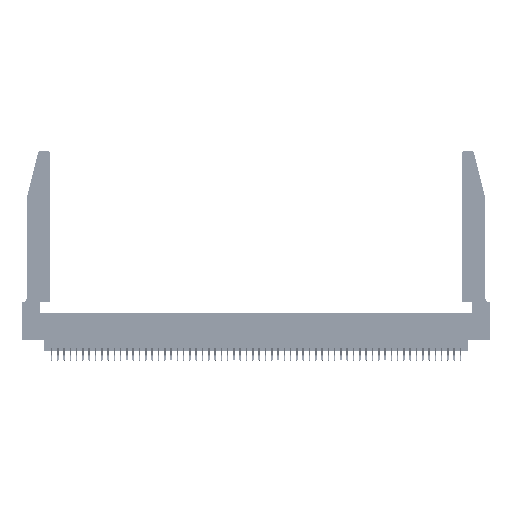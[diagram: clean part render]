
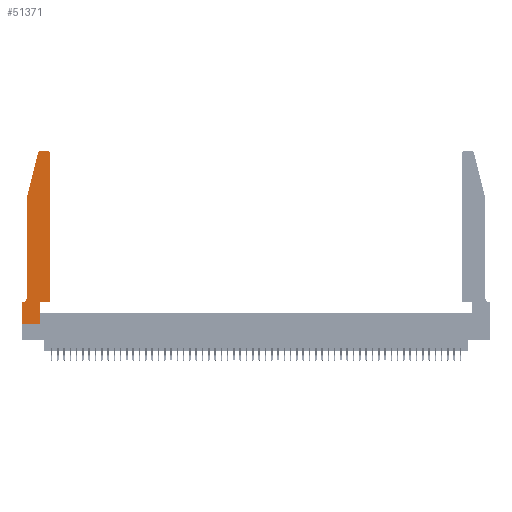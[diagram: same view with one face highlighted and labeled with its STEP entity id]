
A CAD part, top view. The second image highlights one B-rep face of the part: STEP entity #51371.
In plain terms, the highlighted planar face has unit normal (0, 0, 1).
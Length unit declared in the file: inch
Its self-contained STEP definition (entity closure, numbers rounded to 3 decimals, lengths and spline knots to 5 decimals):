
#344 = ORIENTED_EDGE ( 'NONE', *, *, #10502, .T. ) ;
#1664 = CARTESIAN_POINT ( 'NONE',  ( 0.4505, 0.35, 0.37 ) ) ;
#1841 = EDGE_CURVE ( 'NONE', #34388, #30202, #33732, .T. ) ;
#3123 = VECTOR ( 'NONE', #31397, 39.37008 ) ;
#5696 = CIRCLE ( 'NONE', #37060, 0.03 ) ;
#5752 = ORIENTED_EDGE ( 'NONE', *, *, #50961, .T. ) ;
#5858 = VECTOR ( 'NONE', #29512, 39.37008 ) ;
#6128 = CARTESIAN_POINT ( 'NONE',  ( 0.0755, 0.35, 0.37 ) ) ;
#6189 = CARTESIAN_POINT ( 'NONE',  ( 0.25487, 2.72718, 0.37 ) ) ;
#6428 = VERTEX_POINT ( 'NONE', #23156 ) ;
#8055 = DIRECTION ( 'NONE',  ( 1., 0., 0. ) ) ;
#8264 = DIRECTION ( 'NONE',  ( 0., -1., 0. ) ) ;
#8941 = CARTESIAN_POINT ( 'NONE',  ( 0.284, 2.72, 0.37 ) ) ;
#8948 = EDGE_CURVE ( 'NONE', #23391, #43217, #25297, .T. ) ;
#9113 = ORIENTED_EDGE ( 'NONE', *, *, #9363, .T. ) ;
#9363 = EDGE_CURVE ( 'NONE', #19463, #23645, #52215, .T. ) ;
#9889 = CARTESIAN_POINT ( 'NONE',  ( 0.2605, 2.75, 0.37 ) ) ;
#10220 = VECTOR ( 'NONE', #18293, 39.37008 ) ;
#10400 = DIRECTION ( 'NONE',  ( -1., 0., 0. ) ) ;
#10502 = EDGE_CURVE ( 'NONE', #30202, #33000, #11560, .T. ) ;
#11560 = LINE ( 'NONE', #26400, #10220 ) ;
#11642 = EDGE_CURVE ( 'NONE', #33000, #32946, #31454, .T. ) ;
#11741 = ORIENTED_EDGE ( 'NONE', *, *, #11642, .T. ) ;
#12663 = CARTESIAN_POINT ( 'NONE',  ( 0.0055, 0.35, 0.37 ) ) ;
#12953 = VERTEX_POINT ( 'NONE', #25827 ) ;
#13189 = DIRECTION ( 'NONE',  ( 1., 0., 0. ) ) ;
#14351 = VECTOR ( 'NONE', #8055, 39.37008 ) ;
#14960 = ORIENTED_EDGE ( 'NONE', *, *, #40258, .T. ) ;
#15537 = DIRECTION ( 'NONE',  ( 0., 0., 1. ) ) ;
#16232 = CARTESIAN_POINT ( 'NONE',  ( 0., 0., 0.37 ) ) ;
#16848 = VECTOR ( 'NONE', #35021, 39.37008 ) ;
#17118 = DIRECTION ( 'NONE',  ( 0., 0., 1. ) ) ;
#18026 = CARTESIAN_POINT ( 'NONE',  ( 0.0755, 2., 0.37 ) ) ;
#18293 = DIRECTION ( 'NONE',  ( 0., -1., 0. ) ) ;
#18837 = ORIENTED_EDGE ( 'NONE', *, *, #1841, .T. ) ;
#19463 = VERTEX_POINT ( 'NONE', #27011 ) ;
#20140 = CARTESIAN_POINT ( 'NONE',  ( 0.4205, 2.75, 0.37 ) ) ;
#20819 = ORIENTED_EDGE ( 'NONE', *, *, #38945, .T. ) ;
#21031 = CARTESIAN_POINT ( 'NONE',  ( 0., 0.35, 0.37 ) ) ;
#21439 = DIRECTION ( 'NONE',  ( 0., 0., -1. ) ) ;
#23156 = CARTESIAN_POINT ( 'NONE',  ( 0.2865, 0., 0.37 ) ) ;
#23391 = VERTEX_POINT ( 'NONE', #26973 ) ;
#23395 = LINE ( 'NONE', #46493, #33056 ) ;
#23645 = VERTEX_POINT ( 'NONE', #20140 ) ;
#24581 = CARTESIAN_POINT ( 'NONE',  ( 0.4505, 0.35, 0.37 ) ) ;
#24949 = VERTEX_POINT ( 'NONE', #16232 ) ;
#25211 = PLANE ( 'NONE',  #27075 ) ;
#25297 = LINE ( 'NONE', #24581, #14351 ) ;
#25827 = CARTESIAN_POINT ( 'NONE',  ( 0.284, 2.75, 0.37 ) ) ;
#26400 = CARTESIAN_POINT ( 'NONE',  ( 0.0755, 2., 0.37 ) ) ;
#26973 = CARTESIAN_POINT ( 'NONE',  ( 0.2865, 0.35, 0.37 ) ) ;
#27011 = CARTESIAN_POINT ( 'NONE',  ( 0.4505, 2.72, 0.37 ) ) ;
#27075 = AXIS2_PLACEMENT_3D ( 'NONE', #41711, #17118, #45860 ) ;
#27261 = CARTESIAN_POINT ( 'NONE',  ( 0.0755, 2., 0.37 ) ) ;
#27565 = AXIS2_PLACEMENT_3D ( 'NONE', #40151, #15537, #44287 ) ;
#27716 = EDGE_CURVE ( 'NONE', #34018, #24949, #45529, .T. ) ;
#27799 = LINE ( 'NONE', #1664, #16848 ) ;
#28424 = CARTESIAN_POINT ( 'NONE',  ( 0.4505, 0.35, 0.37 ) ) ;
#29176 = ORIENTED_EDGE ( 'NONE', *, *, #27716, .T. ) ;
#29512 = DIRECTION ( 'NONE',  ( 1., 0., 0. ) ) ;
#29517 = EDGE_CURVE ( 'NONE', #23645, #12953, #36391, .T. ) ;
#30202 = VERTEX_POINT ( 'NONE', #18026 ) ;
#30813 = LINE ( 'NONE', #6128, #51331 ) ;
#31397 = DIRECTION ( 'NONE',  ( -0.239, -0.971, 0. ) ) ;
#31454 = CIRCLE ( 'NONE', #35213, 0.07 ) ;
#32946 = VERTEX_POINT ( 'NONE', #12663 ) ;
#33000 = VERTEX_POINT ( 'NONE', #50577 ) ;
#33055 = ORIENTED_EDGE ( 'NONE', *, *, #39697, .T. ) ;
#33056 = VECTOR ( 'NONE', #50604, 39.37008 ) ;
#33732 = LINE ( 'NONE', #27261, #3123 ) ;
#34018 = VERTEX_POINT ( 'NONE', #21031 ) ;
#34034 = EDGE_LOOP ( 'NONE', ( #41317, #14960, #18837, #344, #11741, #5752, #29176, #20819, #33055, #36895, #40744, #9113 ) ) ;
#34388 = VERTEX_POINT ( 'NONE', #6189 ) ;
#34668 = DIRECTION ( 'NONE',  ( -1., 0., 0. ) ) ;
#35021 = DIRECTION ( 'NONE',  ( 0., 1., 0. ) ) ;
#35213 = AXIS2_PLACEMENT_3D ( 'NONE', #46047, #21439, #50171 ) ;
#36391 = LINE ( 'NONE', #9889, #45995 ) ;
#36895 = ORIENTED_EDGE ( 'NONE', *, *, #8948, .T. ) ;
#37060 = AXIS2_PLACEMENT_3D ( 'NONE', #8941, #37830, #13189 ) ;
#37186 = CARTESIAN_POINT ( 'NONE',  ( 0., 0., 0.37 ) ) ;
#37830 = DIRECTION ( 'NONE',  ( 0., 0., 1. ) ) ;
#38902 = LINE ( 'NONE', #46018, #5858 ) ;
#38945 = EDGE_CURVE ( 'NONE', #24949, #6428, #38902, .T. ) ;
#39697 = EDGE_CURVE ( 'NONE', #6428, #23391, #23395, .T. ) ;
#40151 = CARTESIAN_POINT ( 'NONE',  ( 0.4205, 2.72, 0.37 ) ) ;
#40258 = EDGE_CURVE ( 'NONE', #12953, #34388, #5696, .T. ) ;
#40383 = FACE_OUTER_BOUND ( 'NONE', #34034, .T. ) ;
#40744 = ORIENTED_EDGE ( 'NONE', *, *, #48808, .T. ) ;
#41317 = ORIENTED_EDGE ( 'NONE', *, *, #29517, .T. ) ;
#41711 = CARTESIAN_POINT ( 'NONE',  ( 0., 0.35, 0.37 ) ) ;
#42931 = VECTOR ( 'NONE', #8264, 39.37008 ) ;
#43217 = VERTEX_POINT ( 'NONE', #28424 ) ;
#44287 = DIRECTION ( 'NONE',  ( 1., 0., 0. ) ) ;
#45529 = LINE ( 'NONE', #37186, #42931 ) ;
#45860 = DIRECTION ( 'NONE',  ( 1., 0., 0. ) ) ;
#45995 = VECTOR ( 'NONE', #34668, 39.37008 ) ;
#46018 = CARTESIAN_POINT ( 'NONE',  ( 0., 0., 0.37 ) ) ;
#46047 = CARTESIAN_POINT ( 'NONE',  ( 0.0055, 0.42, 0.37 ) ) ;
#46493 = CARTESIAN_POINT ( 'NONE',  ( 0.2865, 0.35, 0.37 ) ) ;
#48808 = EDGE_CURVE ( 'NONE', #43217, #19463, #27799, .T. ) ;
#50171 = DIRECTION ( 'NONE',  ( -1., 0., 0. ) ) ;
#50577 = CARTESIAN_POINT ( 'NONE',  ( 0.0755, 0.42, 0.37 ) ) ;
#50604 = DIRECTION ( 'NONE',  ( 0., 1., 0. ) ) ;
#50961 = EDGE_CURVE ( 'NONE', #32946, #34018, #30813, .T. ) ;
#51331 = VECTOR ( 'NONE', #10400, 39.37008 ) ;
#51371 = ADVANCED_FACE ( 'NONE', ( #40383 ), #25211, .T. ) ;
#52215 = CIRCLE ( 'NONE', #27565, 0.03 ) ;
